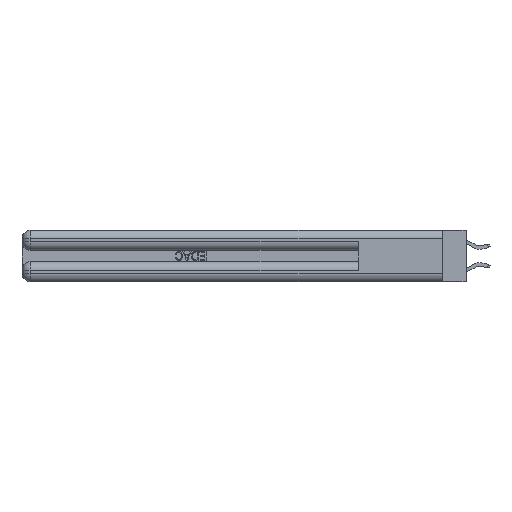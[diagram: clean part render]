
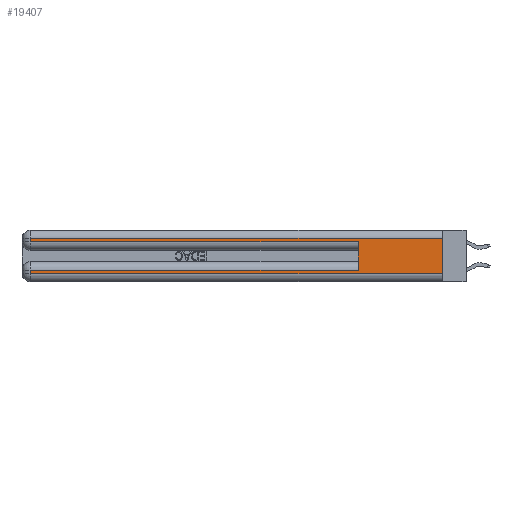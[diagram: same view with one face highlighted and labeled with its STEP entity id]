
A CAD part, left-side view. The second image highlights one B-rep face of the part: STEP entity #19407.
In plain terms, the highlighted planar face has unit normal (-1, 0, 0).
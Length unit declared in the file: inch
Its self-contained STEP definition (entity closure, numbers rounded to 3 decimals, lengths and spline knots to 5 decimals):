
#213 = LINE ( 'NONE', #7765, #28136 ) ;
#237 = VECTOR ( 'NONE', #24829, 39.37008 ) ;
#541 = CARTESIAN_POINT ( 'NONE',  ( 0., 2.94, 0.06 ) ) ;
#1032 = VECTOR ( 'NONE', #32477, 39.37008 ) ;
#1820 = LINE ( 'NONE', #33070, #237 ) ;
#2050 = ORIENTED_EDGE ( 'NONE', *, *, #5859, .T. ) ;
#2152 = CARTESIAN_POINT ( 'NONE',  ( 0., 0., 0.06 ) ) ;
#2302 = VERTEX_POINT ( 'NONE', #541 ) ;
#2625 = DIRECTION ( 'NONE',  ( 0., 0., -1. ) ) ;
#2964 = VECTOR ( 'NONE', #3302, 39.37008 ) ;
#3302 = DIRECTION ( 'NONE',  ( 0., 1., 0. ) ) ;
#4390 = DIRECTION ( 'NONE',  ( 0., 0., -1. ) ) ;
#5794 = VERTEX_POINT ( 'NONE', #2152 ) ;
#5859 = EDGE_CURVE ( 'NONE', #29178, #18533, #14698, .T. ) ;
#5863 = CARTESIAN_POINT ( 'NONE',  ( 0., 0., 0.085 ) ) ;
#5911 = CARTESIAN_POINT ( 'NONE',  ( 0., 2.94, 0.31 ) ) ;
#6670 = DIRECTION ( 'NONE',  ( 0., 0., 1. ) ) ;
#6782 = ORIENTED_EDGE ( 'NONE', *, *, #22358, .F. ) ;
#7765 = CARTESIAN_POINT ( 'NONE',  ( 0., 2.94, 0.37 ) ) ;
#7778 = VECTOR ( 'NONE', #6670, 39.37008 ) ;
#8047 = CARTESIAN_POINT ( 'NONE',  ( 0., 0., 0.31 ) ) ;
#8273 = ORIENTED_EDGE ( 'NONE', *, *, #29807, .T. ) ;
#8656 = EDGE_CURVE ( 'NONE', #31664, #29178, #19473, .T. ) ;
#9300 = LINE ( 'NONE', #17171, #25369 ) ;
#9623 = AXIS2_PLACEMENT_3D ( 'NONE', #31324, #12591, #28565 ) ;
#10002 = ORIENTED_EDGE ( 'NONE', *, *, #12424, .T. ) ;
#10356 = PLANE ( 'NONE',  #9623 ) ;
#11313 = CARTESIAN_POINT ( 'NONE',  ( 0., 0.6, 0.145 ) ) ;
#12424 = EDGE_CURVE ( 'NONE', #32363, #2302, #213, .T. ) ;
#12591 = DIRECTION ( 'NONE',  ( 1., 0., 0. ) ) ;
#12734 = ORIENTED_EDGE ( 'NONE', *, *, #8656, .T. ) ;
#13216 = VERTEX_POINT ( 'NONE', #17996 ) ;
#13764 = ORIENTED_EDGE ( 'NONE', *, *, #32355, .T. ) ;
#14168 = CARTESIAN_POINT ( 'NONE',  ( 0., 0., 0.31 ) ) ;
#14698 = LINE ( 'NONE', #27902, #26805 ) ;
#17061 = DIRECTION ( 'NONE',  ( 0., 1., 0. ) ) ;
#17171 = CARTESIAN_POINT ( 'NONE',  ( 0., 0., 0.285 ) ) ;
#17996 = CARTESIAN_POINT ( 'NONE',  ( 0., 0.6, 0.085 ) ) ;
#18324 = CARTESIAN_POINT ( 'NONE',  ( 0., 2.94, 0.285 ) ) ;
#18533 = VERTEX_POINT ( 'NONE', #18324 ) ;
#18731 = CARTESIAN_POINT ( 'NONE',  ( 0., 0., 0.37 ) ) ;
#19407 = ADVANCED_FACE ( 'NONE', ( #20829 ), #10356, .F. ) ;
#19415 = LINE ( 'NONE', #18731, #1032 ) ;
#19473 = LINE ( 'NONE', #14168, #24247 ) ;
#19969 = CARTESIAN_POINT ( 'NONE',  ( 0., 0.6, 0.285 ) ) ;
#20829 = FACE_OUTER_BOUND ( 'NONE', #29678, .T. ) ;
#22358 = EDGE_CURVE ( 'NONE', #31664, #5794, #19415, .T. ) ;
#23902 = ORIENTED_EDGE ( 'NONE', *, *, #30357, .T. ) ;
#24247 = VECTOR ( 'NONE', #17061, 39.37008 ) ;
#24829 = DIRECTION ( 'NONE',  ( 0., -1., 0. ) ) ;
#24904 = DIRECTION ( 'NONE',  ( 0., -1., 0. ) ) ;
#25369 = VECTOR ( 'NONE', #24904, 39.37008 ) ;
#26805 = VECTOR ( 'NONE', #4390, 39.37008 ) ;
#26817 = ORIENTED_EDGE ( 'NONE', *, *, #28920, .F. ) ;
#27575 = CARTESIAN_POINT ( 'NONE',  ( 0., 2.94, 0.085 ) ) ;
#27902 = CARTESIAN_POINT ( 'NONE',  ( 0., 2.94, 0.37 ) ) ;
#28136 = VECTOR ( 'NONE', #2625, 39.37008 ) ;
#28565 = DIRECTION ( 'NONE',  ( 0., 0., -1. ) ) ;
#28920 = EDGE_CURVE ( 'NONE', #13216, #32797, #30045, .T. ) ;
#29178 = VERTEX_POINT ( 'NONE', #5911 ) ;
#29392 = LINE ( 'NONE', #5863, #2964 ) ;
#29678 = EDGE_LOOP ( 'NONE', ( #6782, #12734, #2050, #8273, #26817, #23902, #10002, #13764 ) ) ;
#29807 = EDGE_CURVE ( 'NONE', #18533, #32797, #9300, .T. ) ;
#30045 = LINE ( 'NONE', #11313, #7778 ) ;
#30357 = EDGE_CURVE ( 'NONE', #13216, #32363, #29392, .T. ) ;
#31324 = CARTESIAN_POINT ( 'NONE',  ( 0., 0., 0.37 ) ) ;
#31664 = VERTEX_POINT ( 'NONE', #8047 ) ;
#32355 = EDGE_CURVE ( 'NONE', #2302, #5794, #1820, .T. ) ;
#32363 = VERTEX_POINT ( 'NONE', #27575 ) ;
#32477 = DIRECTION ( 'NONE',  ( 0., 0., -1. ) ) ;
#32797 = VERTEX_POINT ( 'NONE', #19969 ) ;
#33070 = CARTESIAN_POINT ( 'NONE',  ( 0., 0., 0.06 ) ) ;
